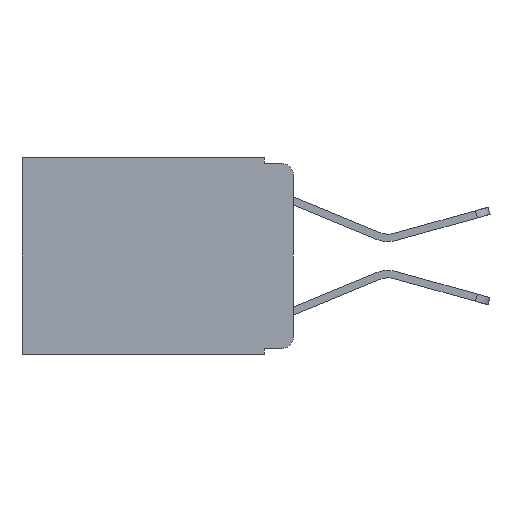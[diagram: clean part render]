
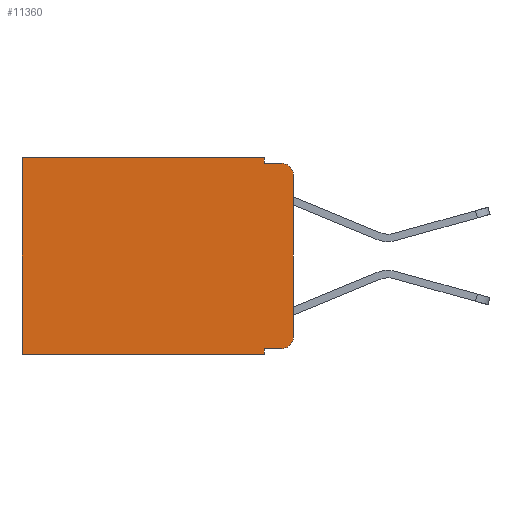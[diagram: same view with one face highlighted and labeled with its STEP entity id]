
A CAD part, left-side view. The second image highlights one B-rep face of the part: STEP entity #11360.
In plain terms, the highlighted planar face has unit normal (-1, 0, 0).
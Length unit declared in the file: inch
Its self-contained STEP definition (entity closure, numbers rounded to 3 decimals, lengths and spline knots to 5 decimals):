
#462 = VECTOR ( 'NONE', #2925, 39.37008 ) ;
#508 = ORIENTED_EDGE ( 'NONE', *, *, #8121, .T. ) ;
#622 = CARTESIAN_POINT ( 'NONE',  ( 0.298, 0.051, -0.01 ) ) ;
#795 = ORIENTED_EDGE ( 'NONE', *, *, #12105, .T. ) ;
#1169 = VERTEX_POINT ( 'NONE', #16036 ) ;
#1245 = CARTESIAN_POINT ( 'NONE',  ( 0.298, 0.051, 0. ) ) ;
#1387 = CARTESIAN_POINT ( 'NONE',  ( 0.298, 0., 0. ) ) ;
#1592 = VERTEX_POINT ( 'NONE', #18318 ) ;
#1617 = EDGE_CURVE ( 'NONE', #17788, #12604, #9861, .T. ) ;
#1956 = LINE ( 'NONE', #1387, #462 ) ;
#2026 = CARTESIAN_POINT ( 'NONE',  ( 0.298, 0.473, -0.343 ) ) ;
#2086 = LINE ( 'NONE', #10875, #13427 ) ;
#2150 = CARTESIAN_POINT ( 'NONE',  ( 0.298, 0., -0.03 ) ) ;
#2199 = DIRECTION ( 'NONE',  ( 0., -1., 0. ) ) ;
#2230 = VECTOR ( 'NONE', #2199, 39.37008 ) ;
#2457 = LINE ( 'NONE', #5258, #13804 ) ;
#2710 = PLANE ( 'NONE',  #7686 ) ;
#2844 = CARTESIAN_POINT ( 'NONE',  ( 0.298, 0., 0. ) ) ;
#2925 = DIRECTION ( 'NONE',  ( 0., 1., 0. ) ) ;
#2948 = ORIENTED_EDGE ( 'NONE', *, *, #15395, .T. ) ;
#3276 = CARTESIAN_POINT ( 'NONE',  ( 0.298, 0.051, 0. ) ) ;
#3923 = ORIENTED_EDGE ( 'NONE', *, *, #1617, .T. ) ;
#4395 = ORIENTED_EDGE ( 'NONE', *, *, #15874, .F. ) ;
#4747 = CARTESIAN_POINT ( 'NONE',  ( 0.298, 0.473, 0. ) ) ;
#5162 = EDGE_CURVE ( 'NONE', #1169, #1592, #18600, .T. ) ;
#5258 = CARTESIAN_POINT ( 'NONE',  ( 0.298, 0., -0.343 ) ) ;
#5764 = ORIENTED_EDGE ( 'NONE', *, *, #12107, .F. ) ;
#5873 = DIRECTION ( 'NONE',  ( 0., 0., -1. ) ) ;
#6037 = VERTEX_POINT ( 'NONE', #3276 ) ;
#6403 = CARTESIAN_POINT ( 'NONE',  ( 0.298, 0.02, -0.01 ) ) ;
#6421 = ORIENTED_EDGE ( 'NONE', *, *, #5162, .F. ) ;
#6734 = DIRECTION ( 'NONE',  ( -1., 0., 0. ) ) ;
#6739 = CARTESIAN_POINT ( 'NONE',  ( 0.298, 0.02, -0.03 ) ) ;
#6955 = AXIS2_PLACEMENT_3D ( 'NONE', #6739, #17017, #8219 ) ;
#7686 = AXIS2_PLACEMENT_3D ( 'NONE', #2844, #14659, #5873 ) ;
#8121 = EDGE_CURVE ( 'NONE', #9012, #14499, #12352, .T. ) ;
#8219 = DIRECTION ( 'NONE',  ( 0., 0., -1. ) ) ;
#9012 = VERTEX_POINT ( 'NONE', #11547 ) ;
#9214 = DIRECTION ( 'NONE',  ( 0., 0., -1. ) ) ;
#9272 = VECTOR ( 'NONE', #15357, 39.37008 ) ;
#9391 = DIRECTION ( 'NONE',  ( 0., 0., -1. ) ) ;
#9664 = ORIENTED_EDGE ( 'NONE', *, *, #9882, .F. ) ;
#9861 = CIRCLE ( 'NONE', #6955, 0.02 ) ;
#9882 = EDGE_CURVE ( 'NONE', #6037, #12277, #13177, .T. ) ;
#10128 = CARTESIAN_POINT ( 'NONE',  ( 0.298, 0.051, -0.01 ) ) ;
#10231 = DIRECTION ( 'NONE',  ( 0., 0., -1. ) ) ;
#10320 = EDGE_LOOP ( 'NONE', ( #12072, #3923, #4395, #9664, #12866, #508, #5764, #6421, #2948, #795 ) ) ;
#10401 = CIRCLE ( 'NONE', #16811, 0.02 ) ;
#10478 = CARTESIAN_POINT ( 'NONE',  ( 0.298, 0., -0.313 ) ) ;
#10875 = CARTESIAN_POINT ( 'NONE',  ( 0.298, 0., 0. ) ) ;
#11074 = FACE_OUTER_BOUND ( 'NONE', #10320, .T. ) ;
#11116 = DIRECTION ( 'NONE',  ( 0., 1., 0. ) ) ;
#11360 = ADVANCED_FACE ( 'NONE', ( #11074 ), #2710, .F. ) ;
#11547 = CARTESIAN_POINT ( 'NONE',  ( 0.298, 0.473, 0. ) ) ;
#11891 = VECTOR ( 'NONE', #9214, 39.37008 ) ;
#12072 = ORIENTED_EDGE ( 'NONE', *, *, #13908, .F. ) ;
#12105 = EDGE_CURVE ( 'NONE', #18400, #13091, #10401, .T. ) ;
#12107 = EDGE_CURVE ( 'NONE', #1592, #14499, #2457, .T. ) ;
#12277 = VERTEX_POINT ( 'NONE', #10128 ) ;
#12352 = LINE ( 'NONE', #4747, #11891 ) ;
#12515 = CARTESIAN_POINT ( 'NONE',  ( 0.298, 0.02, -0.333 ) ) ;
#12604 = VERTEX_POINT ( 'NONE', #6403 ) ;
#12866 = ORIENTED_EDGE ( 'NONE', *, *, #13041, .T. ) ;
#13041 = EDGE_CURVE ( 'NONE', #6037, #9012, #1956, .T. ) ;
#13091 = VERTEX_POINT ( 'NONE', #10478 ) ;
#13177 = LINE ( 'NONE', #15287, #9272 ) ;
#13427 = VECTOR ( 'NONE', #9391, 39.37008 ) ;
#13804 = VECTOR ( 'NONE', #11116, 39.37008 ) ;
#13908 = EDGE_CURVE ( 'NONE', #17788, #13091, #2086, .T. ) ;
#14181 = DIRECTION ( 'NONE',  ( 0., -1., 0. ) ) ;
#14499 = VERTEX_POINT ( 'NONE', #2026 ) ;
#14659 = DIRECTION ( 'NONE',  ( 1., 0., 0. ) ) ;
#14983 = VECTOR ( 'NONE', #14181, 39.37008 ) ;
#15287 = CARTESIAN_POINT ( 'NONE',  ( 0.298, 0.051, 0. ) ) ;
#15357 = DIRECTION ( 'NONE',  ( 0., 0., -1. ) ) ;
#15395 = EDGE_CURVE ( 'NONE', #1169, #18400, #18800, .T. ) ;
#15548 = CARTESIAN_POINT ( 'NONE',  ( 0.298, 0.02, -0.313 ) ) ;
#15647 = CARTESIAN_POINT ( 'NONE',  ( 0.298, 0.051, -0.333 ) ) ;
#15693 = VECTOR ( 'NONE', #10231, 39.37008 ) ;
#15874 = EDGE_CURVE ( 'NONE', #12277, #12604, #18781, .T. ) ;
#16036 = CARTESIAN_POINT ( 'NONE',  ( 0.298, 0.051, -0.333 ) ) ;
#16811 = AXIS2_PLACEMENT_3D ( 'NONE', #15548, #6734, #17013 ) ;
#17013 = DIRECTION ( 'NONE',  ( 0., 0., -1. ) ) ;
#17017 = DIRECTION ( 'NONE',  ( -1., 0., 0. ) ) ;
#17788 = VERTEX_POINT ( 'NONE', #2150 ) ;
#18318 = CARTESIAN_POINT ( 'NONE',  ( 0.298, 0.051, -0.343 ) ) ;
#18400 = VERTEX_POINT ( 'NONE', #12515 ) ;
#18600 = LINE ( 'NONE', #1245, #15693 ) ;
#18781 = LINE ( 'NONE', #622, #2230 ) ;
#18800 = LINE ( 'NONE', #15647, #14983 ) ;
